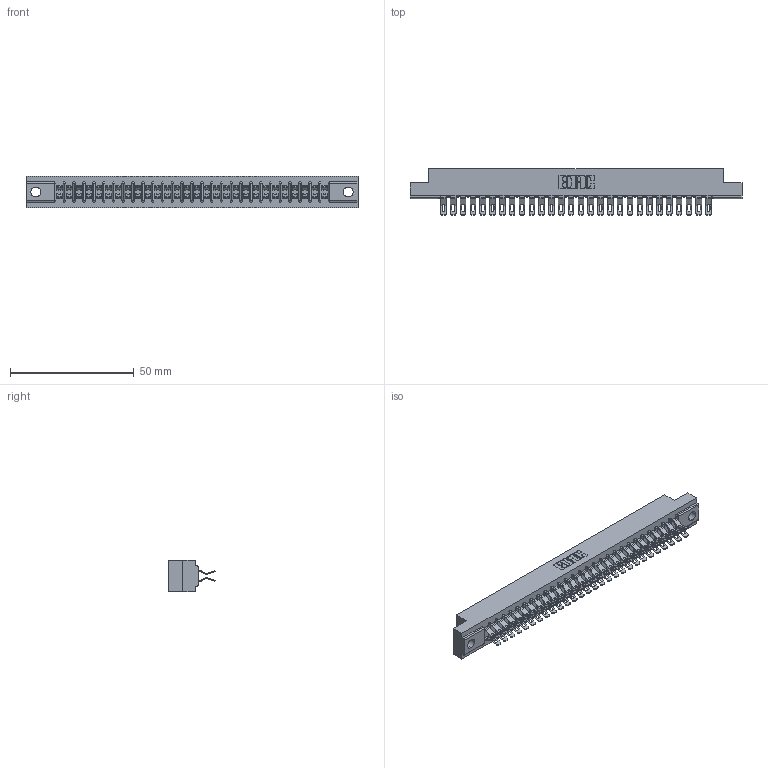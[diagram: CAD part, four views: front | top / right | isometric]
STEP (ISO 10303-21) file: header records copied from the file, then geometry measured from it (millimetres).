
FILE_DESCRIPTION (( 'STEP AP203' ), '1' );
FILE_NAME ('307-056-555-204.STEP', '2019-09-06T13:41:01', ( '' ), ( '' ), 'SwSTEP 2.0', 'SolidWorks 2016', '' );
FILE_SCHEMA (( 'CONFIG_CONTROL_DESIGN' ));
Length unit declared in the file: inch
Products named in the file (3): 307 Part_.156 Dia Mounting Holes; 307-056-555-204; 307-290-001_555
Assembly tree (57 placements, depth 2):
  307-056-555-204
    307 Part_.156 Dia Mounting Holes
    307-290-001_555  x56
Bounding box: 133.96 x 18.75 x 12.7 mm (x, y, z)
Volume: 14206.7 mm3; surface area: 17859.7 mm2
Topology: 57 solids, 57 shells, 3577 faces, 10495 edges, 6842 vertices
Faces by surface type: plane 1988, cylinder 1531, sphere 58
Entity records: 27581 total; most frequent: CARTESIAN_POINT 4526, ORIENTED_EDGE 4484, DIRECTION 4438, EDGE_CURVE 2242, VECTOR 1710, LINE 1710, VERTEX_POINT 1452, AXIS2_PLACEMENT_3D 1364
